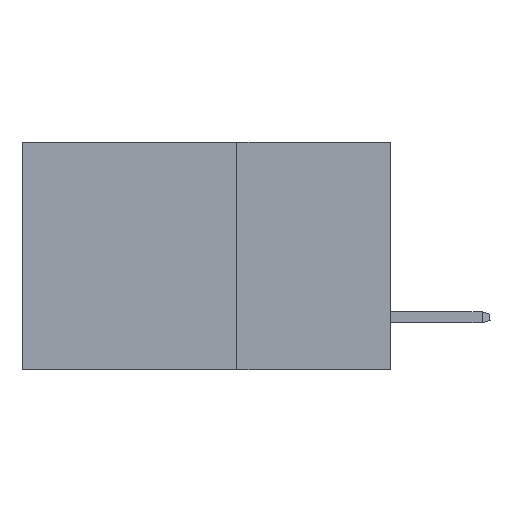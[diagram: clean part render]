
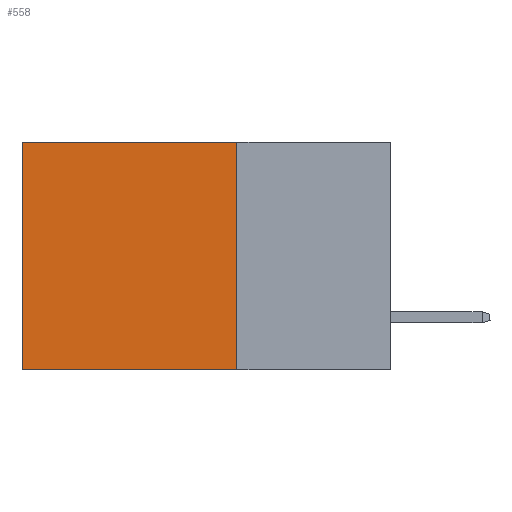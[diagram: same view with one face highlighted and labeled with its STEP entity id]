
A CAD part, left-side view. The second image highlights one B-rep face of the part: STEP entity #558.
In plain terms, the highlighted planar face has unit normal (-1, 0, 0).
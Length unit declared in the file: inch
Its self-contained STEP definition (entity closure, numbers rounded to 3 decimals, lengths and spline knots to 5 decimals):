
#558 = ADVANCED_FACE ( 'NONE', ( #1209 ), #735, .F. ) ;
#596 = EDGE_CURVE ( 'NONE', #8493, #6707, #4497, .T. ) ;
#735 = PLANE ( 'NONE',  #1290 ) ;
#750 = CARTESIAN_POINT ( 'NONE',  ( 0.2875, 0.25, -0.37 ) ) ;
#785 = VECTOR ( 'NONE', #3119, 39.37008 ) ;
#876 = VECTOR ( 'NONE', #3916, 39.37008 ) ;
#1209 = FACE_OUTER_BOUND ( 'NONE', #4385, .T. ) ;
#1265 = EDGE_CURVE ( 'NONE', #5975, #6707, #6285, .T. ) ;
#1290 = AXIS2_PLACEMENT_3D ( 'NONE', #1614, #3959, #5468 ) ;
#1614 = CARTESIAN_POINT ( 'NONE',  ( 0.2875, 0.25, 0. ) ) ;
#2793 = VECTOR ( 'NONE', #8113, 39.37008 ) ;
#2965 = CARTESIAN_POINT ( 'NONE',  ( 0.2875, 0.6, -0.37 ) ) ;
#3119 = DIRECTION ( 'NONE',  ( 0., 1., 0. ) ) ;
#3217 = EDGE_CURVE ( 'NONE', #8271, #8493, #6439, .T. ) ;
#3916 = DIRECTION ( 'NONE',  ( 0., 0., -1. ) ) ;
#3959 = DIRECTION ( 'NONE',  ( 1., 0., 0. ) ) ;
#4001 = CARTESIAN_POINT ( 'NONE',  ( 0.2875, 0.6, 0. ) ) ;
#4268 = ORIENTED_EDGE ( 'NONE', *, *, #1265, .T. ) ;
#4374 = ORIENTED_EDGE ( 'NONE', *, *, #6119, .T. ) ;
#4385 = EDGE_LOOP ( 'NONE', ( #4268, #8172, #8603, #4374 ) ) ;
#4497 = LINE ( 'NONE', #750, #785 ) ;
#4528 = VECTOR ( 'NONE', #4816, 39.37008 ) ;
#4639 = LINE ( 'NONE', #8784, #2793 ) ;
#4688 = CARTESIAN_POINT ( 'NONE',  ( 0.2875, 0.6, 0. ) ) ;
#4816 = DIRECTION ( 'NONE',  ( 0., 0., -1. ) ) ;
#5136 = CARTESIAN_POINT ( 'NONE',  ( 0.2875, 0.25, 0. ) ) ;
#5468 = DIRECTION ( 'NONE',  ( 0., 0., -1. ) ) ;
#5975 = VERTEX_POINT ( 'NONE', #4688 ) ;
#6119 = EDGE_CURVE ( 'NONE', #8271, #5975, #4639, .T. ) ;
#6285 = LINE ( 'NONE', #4001, #876 ) ;
#6439 = LINE ( 'NONE', #5136, #4528 ) ;
#6707 = VERTEX_POINT ( 'NONE', #2965 ) ;
#7161 = CARTESIAN_POINT ( 'NONE',  ( 0.2875, 0.25, -0.37 ) ) ;
#8113 = DIRECTION ( 'NONE',  ( 0., 1., 0. ) ) ;
#8172 = ORIENTED_EDGE ( 'NONE', *, *, #596, .F. ) ;
#8271 = VERTEX_POINT ( 'NONE', #8296 ) ;
#8296 = CARTESIAN_POINT ( 'NONE',  ( 0.2875, 0.25, 0. ) ) ;
#8493 = VERTEX_POINT ( 'NONE', #7161 ) ;
#8603 = ORIENTED_EDGE ( 'NONE', *, *, #3217, .F. ) ;
#8784 = CARTESIAN_POINT ( 'NONE',  ( 0.2875, 0.25, 0. ) ) ;
